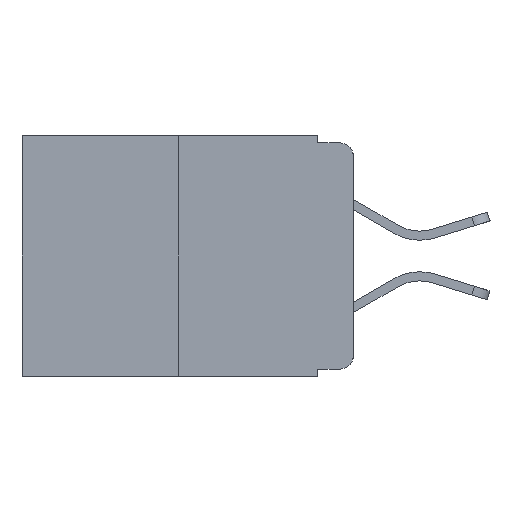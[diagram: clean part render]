
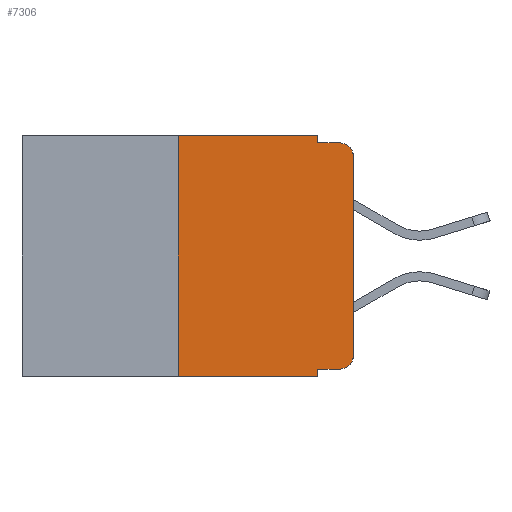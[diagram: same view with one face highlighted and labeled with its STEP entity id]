
A CAD part, left-side view. The second image highlights one B-rep face of the part: STEP entity #7306.
In plain terms, the highlighted planar face has unit normal (-1, 0, 0).
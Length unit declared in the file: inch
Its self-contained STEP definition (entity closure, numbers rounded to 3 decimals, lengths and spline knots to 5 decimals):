
#78 = CARTESIAN_POINT ( 'NONE',  ( 0., 0.051, -0.01 ) ) ;
#259 = ORIENTED_EDGE ( 'NONE', *, *, #14623, .T. ) ;
#307 = EDGE_CURVE ( 'NONE', #11743, #13441, #6506, .T. ) ;
#527 = ORIENTED_EDGE ( 'NONE', *, *, #6619, .T. ) ;
#1634 = VECTOR ( 'NONE', #15400, 39.37008 ) ;
#1645 = LINE ( 'NONE', #13350, #9400 ) ;
#1967 = AXIS2_PLACEMENT_3D ( 'NONE', #12991, #3782, #14478 ) ;
#2079 = VECTOR ( 'NONE', #2199, 39.37008 ) ;
#2199 = DIRECTION ( 'NONE',  ( 0., 0., -1. ) ) ;
#2224 = DIRECTION ( 'NONE',  ( 0., 0., -1. ) ) ;
#2338 = ORIENTED_EDGE ( 'NONE', *, *, #14390, .F. ) ;
#2366 = CARTESIAN_POINT ( 'NONE',  ( 0., 0.473, 0. ) ) ;
#2408 = VECTOR ( 'NONE', #4057, 39.37008 ) ;
#2463 = EDGE_CURVE ( 'NONE', #4548, #8950, #6661, .T. ) ;
#2507 = VERTEX_POINT ( 'NONE', #15732 ) ;
#3335 = EDGE_CURVE ( 'NONE', #16324, #4676, #16164, .T. ) ;
#3558 = VERTEX_POINT ( 'NONE', #11988 ) ;
#3782 = DIRECTION ( 'NONE',  ( -1., 0., 0. ) ) ;
#4057 = DIRECTION ( 'NONE',  ( 0., 0., 1. ) ) ;
#4548 = VERTEX_POINT ( 'NONE', #19848 ) ;
#4676 = VERTEX_POINT ( 'NONE', #11066 ) ;
#5227 = EDGE_CURVE ( 'NONE', #2507, #4548, #9478, .T. ) ;
#5452 = CARTESIAN_POINT ( 'NONE',  ( 0., 0.473, -0.343 ) ) ;
#5479 = DIRECTION ( 'NONE',  ( 0., 0., -1. ) ) ;
#6093 = LINE ( 'NONE', #11490, #17737 ) ;
#6302 = VERTEX_POINT ( 'NONE', #12173 ) ;
#6506 = LINE ( 'NONE', #8336, #2408 ) ;
#6619 = EDGE_CURVE ( 'NONE', #13441, #3558, #15368, .T. ) ;
#6661 = LINE ( 'NONE', #18079, #2079 ) ;
#6686 = CARTESIAN_POINT ( 'NONE',  ( 0., 0.051, -0.333 ) ) ;
#7306 = ADVANCED_FACE ( 'NONE', ( #11058 ), #13160, .F. ) ;
#7639 = EDGE_CURVE ( 'NONE', #8950, #3558, #13951, .T. ) ;
#7862 = CARTESIAN_POINT ( 'NONE',  ( 0., 0.02, -0.313 ) ) ;
#7943 = EDGE_CURVE ( 'NONE', #6302, #11451, #12754, .T. ) ;
#8336 = CARTESIAN_POINT ( 'NONE',  ( 0., 0., 0. ) ) ;
#8445 = AXIS2_PLACEMENT_3D ( 'NONE', #7862, #18430, #9421 ) ;
#8950 = VERTEX_POINT ( 'NONE', #78 ) ;
#9400 = VECTOR ( 'NONE', #14884, 39.37008 ) ;
#9421 = DIRECTION ( 'NONE',  ( 0., 0., -1. ) ) ;
#9478 = LINE ( 'NONE', #15484, #17043 ) ;
#9631 = CIRCLE ( 'NONE', #8445, 0.02 ) ;
#10543 = ORIENTED_EDGE ( 'NONE', *, *, #7943, .T. ) ;
#10616 = CARTESIAN_POINT ( 'NONE',  ( 0., 0., -0.313 ) ) ;
#10918 = EDGE_CURVE ( 'NONE', #16324, #11451, #6093, .T. ) ;
#11058 = FACE_OUTER_BOUND ( 'NONE', #15401, .T. ) ;
#11066 = CARTESIAN_POINT ( 'NONE',  ( 0., 0.02, -0.333 ) ) ;
#11451 = VERTEX_POINT ( 'NONE', #17398 ) ;
#11490 = CARTESIAN_POINT ( 'NONE',  ( 0., 0.051, 0. ) ) ;
#11743 = VERTEX_POINT ( 'NONE', #10616 ) ;
#11988 = CARTESIAN_POINT ( 'NONE',  ( 0., 0.02, -0.01 ) ) ;
#12173 = CARTESIAN_POINT ( 'NONE',  ( 0., 0.25, -0.343 ) ) ;
#12206 = ORIENTED_EDGE ( 'NONE', *, *, #2463, .F. ) ;
#12628 = CARTESIAN_POINT ( 'NONE',  ( 0., 0., -0.03 ) ) ;
#12754 = LINE ( 'NONE', #5452, #13250 ) ;
#12991 = CARTESIAN_POINT ( 'NONE',  ( 0., 0.02, -0.03 ) ) ;
#13160 = PLANE ( 'NONE',  #13611 ) ;
#13250 = VECTOR ( 'NONE', #14616, 39.37008 ) ;
#13350 = CARTESIAN_POINT ( 'NONE',  ( 0., 0.25, 0. ) ) ;
#13441 = VERTEX_POINT ( 'NONE', #12628 ) ;
#13611 = AXIS2_PLACEMENT_3D ( 'NONE', #2366, #14641, #5479 ) ;
#13951 = LINE ( 'NONE', #19801, #1634 ) ;
#14390 = EDGE_CURVE ( 'NONE', #6302, #2507, #1645, .T. ) ;
#14478 = DIRECTION ( 'NONE',  ( 0., 0., -1. ) ) ;
#14616 = DIRECTION ( 'NONE',  ( 0., -1., 0. ) ) ;
#14623 = EDGE_CURVE ( 'NONE', #4676, #11743, #9631, .T. ) ;
#14641 = DIRECTION ( 'NONE',  ( 1., 0., 0. ) ) ;
#14884 = DIRECTION ( 'NONE',  ( 0., 0., 1. ) ) ;
#15368 = CIRCLE ( 'NONE', #1967, 0.02 ) ;
#15400 = DIRECTION ( 'NONE',  ( 0., -1., 0. ) ) ;
#15401 = EDGE_LOOP ( 'NONE', ( #19642, #527, #18746, #12206, #17595, #2338, #10543, #19637, #16181, #259 ) ) ;
#15484 = CARTESIAN_POINT ( 'NONE',  ( 0., 0.473, 0. ) ) ;
#15732 = CARTESIAN_POINT ( 'NONE',  ( 0., 0.25, 0. ) ) ;
#16164 = LINE ( 'NONE', #6686, #18701 ) ;
#16181 = ORIENTED_EDGE ( 'NONE', *, *, #3335, .T. ) ;
#16324 = VERTEX_POINT ( 'NONE', #18693 ) ;
#17001 = DIRECTION ( 'NONE',  ( 0., -1., 0. ) ) ;
#17043 = VECTOR ( 'NONE', #17001, 39.37008 ) ;
#17398 = CARTESIAN_POINT ( 'NONE',  ( 0., 0.051, -0.343 ) ) ;
#17595 = ORIENTED_EDGE ( 'NONE', *, *, #5227, .F. ) ;
#17737 = VECTOR ( 'NONE', #2224, 39.37008 ) ;
#18079 = CARTESIAN_POINT ( 'NONE',  ( 0., 0.051, 0. ) ) ;
#18430 = DIRECTION ( 'NONE',  ( -1., 0., 0. ) ) ;
#18693 = CARTESIAN_POINT ( 'NONE',  ( 0., 0.051, -0.333 ) ) ;
#18701 = VECTOR ( 'NONE', #19717, 39.37008 ) ;
#18746 = ORIENTED_EDGE ( 'NONE', *, *, #7639, .F. ) ;
#19637 = ORIENTED_EDGE ( 'NONE', *, *, #10918, .F. ) ;
#19642 = ORIENTED_EDGE ( 'NONE', *, *, #307, .T. ) ;
#19717 = DIRECTION ( 'NONE',  ( 0., -1., 0. ) ) ;
#19801 = CARTESIAN_POINT ( 'NONE',  ( 0., 0.051, -0.01 ) ) ;
#19848 = CARTESIAN_POINT ( 'NONE',  ( 0., 0.051, 0. ) ) ;
